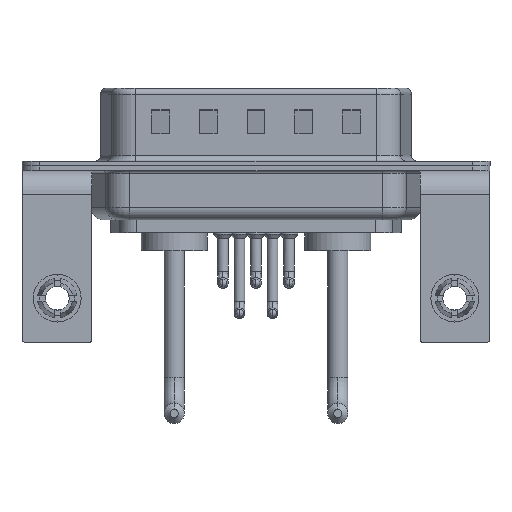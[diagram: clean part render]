
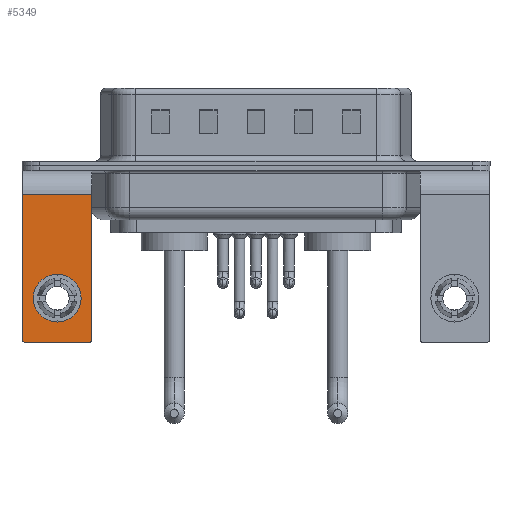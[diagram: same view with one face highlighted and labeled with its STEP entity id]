
A CAD part, front view. The second image highlights one B-rep face of the part: STEP entity #5349.
In plain terms, the highlighted planar face has unit normal (0, -1, 0).
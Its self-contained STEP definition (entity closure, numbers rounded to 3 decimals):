
#20 = VECTOR ( 'NONE', #5921, 1000. ) ;
#798 = CARTESIAN_POINT ( 'NONE',  ( 2.9, -6.25, -2.4 ) ) ;
#883 = VERTEX_POINT ( 'NONE', #15094 ) ;
#1487 = DIRECTION ( 'NONE',  ( 0., 0., 1. ) ) ;
#1555 = DIRECTION ( 'NONE',  ( 0., 0., 1. ) ) ;
#1979 = LINE ( 'NONE', #7727, #20 ) ;
#2088 = ORIENTED_EDGE ( 'NONE', *, *, #6716, .T. ) ;
#2106 = CARTESIAN_POINT ( 'NONE',  ( 2.9, -6.25, -14.8 ) ) ;
#2457 = ORIENTED_EDGE ( 'NONE', *, *, #6031, .T. ) ;
#2929 = DIRECTION ( 'NONE',  ( 0., -1., 0. ) ) ;
#2950 = DIRECTION ( 'NONE',  ( 0., 0., 1. ) ) ;
#2964 = ORIENTED_EDGE ( 'NONE', *, *, #12730, .T. ) ;
#4126 = EDGE_CURVE ( 'NONE', #15058, #19484, #11957, .T. ) ;
#4649 = EDGE_LOOP ( 'NONE', ( #2964, #17490, #8365, #11468, #14675, #2088 ) ) ;
#4917 = AXIS2_PLACEMENT_3D ( 'NONE', #13204, #9195, #7426 ) ;
#5349 = ADVANCED_FACE ( 'NONE', ( #21901, #9768 ), #14740, .F. ) ;
#5570 = LINE ( 'NONE', #2106, #12063 ) ;
#5921 = DIRECTION ( 'NONE',  ( -1., 0., 0. ) ) ;
#6031 = EDGE_CURVE ( 'NONE', #11225, #16553, #15951, .T. ) ;
#6227 = EDGE_LOOP ( 'NONE', ( #20893, #2457 ) ) ;
#6716 = EDGE_CURVE ( 'NONE', #13301, #883, #1979, .T. ) ;
#7186 = CARTESIAN_POINT ( 'NONE',  ( -2.9, -6.25, -2.4 ) ) ;
#7426 = DIRECTION ( 'NONE',  ( 0., 0., 1. ) ) ;
#7727 = CARTESIAN_POINT ( 'NONE',  ( 2.9, -6.25, -2.4 ) ) ;
#8365 = ORIENTED_EDGE ( 'NONE', *, *, #22957, .F. ) ;
#8674 = CARTESIAN_POINT ( 'NONE',  ( 0., -6.25, -13.07 ) ) ;
#8946 = CARTESIAN_POINT ( 'NONE',  ( 2.65, -6.25, -14.55 ) ) ;
#8986 = VECTOR ( 'NONE', #18318, 1000. ) ;
#9195 = DIRECTION ( 'NONE',  ( 0., 1., 0. ) ) ;
#9244 = CIRCLE ( 'NONE', #14517, 0.25 ) ;
#9303 = VECTOR ( 'NONE', #13648, 1000. ) ;
#9751 = CARTESIAN_POINT ( 'NONE',  ( 2.9, -6.25, -14.55 ) ) ;
#9768 = FACE_OUTER_BOUND ( 'NONE', #4649, .T. ) ;
#10831 = DIRECTION ( 'NONE',  ( 0., -1., 0. ) ) ;
#11202 = DIRECTION ( 'NONE',  ( 0., 0., 1. ) ) ;
#11225 = VERTEX_POINT ( 'NONE', #20452 ) ;
#11468 = ORIENTED_EDGE ( 'NONE', *, *, #4126, .T. ) ;
#11472 = EDGE_CURVE ( 'NONE', #13301, #19484, #13886, .T. ) ;
#11774 = AXIS2_PLACEMENT_3D ( 'NONE', #18873, #19228, #2950 ) ;
#11957 = CIRCLE ( 'NONE', #18405, 0.25 ) ;
#12063 = VECTOR ( 'NONE', #21720, 1000. ) ;
#12730 = EDGE_CURVE ( 'NONE', #883, #22783, #16063, .T. ) ;
#13036 = CARTESIAN_POINT ( 'NONE',  ( -2.65, -6.25, -14.8 ) ) ;
#13204 = CARTESIAN_POINT ( 'NONE',  ( 0., -6.25, -11.07 ) ) ;
#13213 = VERTEX_POINT ( 'NONE', #13036 ) ;
#13301 = VERTEX_POINT ( 'NONE', #798 ) ;
#13539 = EDGE_CURVE ( 'NONE', #22783, #13213, #9244, .T. ) ;
#13590 = CIRCLE ( 'NONE', #4917, 2. ) ;
#13648 = DIRECTION ( 'NONE',  ( 0., 0., -1. ) ) ;
#13886 = LINE ( 'NONE', #17460, #9303 ) ;
#14517 = AXIS2_PLACEMENT_3D ( 'NONE', #17766, #2929, #1487 ) ;
#14675 = ORIENTED_EDGE ( 'NONE', *, *, #11472, .F. ) ;
#14740 = PLANE ( 'NONE',  #15937 ) ;
#15058 = VERTEX_POINT ( 'NONE', #16134 ) ;
#15094 = CARTESIAN_POINT ( 'NONE',  ( -2.9, -6.25, -2.4 ) ) ;
#15937 = AXIS2_PLACEMENT_3D ( 'NONE', #20575, #20460, #11202 ) ;
#15951 = CIRCLE ( 'NONE', #11774, 2. ) ;
#16063 = LINE ( 'NONE', #7186, #8986 ) ;
#16134 = CARTESIAN_POINT ( 'NONE',  ( 2.65, -6.25, -14.8 ) ) ;
#16553 = VERTEX_POINT ( 'NONE', #8674 ) ;
#17460 = CARTESIAN_POINT ( 'NONE',  ( 2.9, -6.25, -2.4 ) ) ;
#17490 = ORIENTED_EDGE ( 'NONE', *, *, #13539, .T. ) ;
#17560 = CARTESIAN_POINT ( 'NONE',  ( -2.9, -6.25, -14.55 ) ) ;
#17766 = CARTESIAN_POINT ( 'NONE',  ( -2.65, -6.25, -14.55 ) ) ;
#18318 = DIRECTION ( 'NONE',  ( 0., 0., -1. ) ) ;
#18405 = AXIS2_PLACEMENT_3D ( 'NONE', #8946, #10831, #1555 ) ;
#18822 = EDGE_CURVE ( 'NONE', #16553, #11225, #13590, .T. ) ;
#18873 = CARTESIAN_POINT ( 'NONE',  ( 0., -6.25, -11.07 ) ) ;
#19228 = DIRECTION ( 'NONE',  ( 0., 1., 0. ) ) ;
#19484 = VERTEX_POINT ( 'NONE', #9751 ) ;
#20452 = CARTESIAN_POINT ( 'NONE',  ( 0., -6.25, -9.07 ) ) ;
#20460 = DIRECTION ( 'NONE',  ( 0., 1., 0. ) ) ;
#20575 = CARTESIAN_POINT ( 'NONE',  ( 2.9, -6.25, -2.4 ) ) ;
#20893 = ORIENTED_EDGE ( 'NONE', *, *, #18822, .T. ) ;
#21720 = DIRECTION ( 'NONE',  ( -1., 0., 0. ) ) ;
#21901 = FACE_BOUND ( 'NONE', #6227, .T. ) ;
#22783 = VERTEX_POINT ( 'NONE', #17560 ) ;
#22957 = EDGE_CURVE ( 'NONE', #15058, #13213, #5570, .T. ) ;
